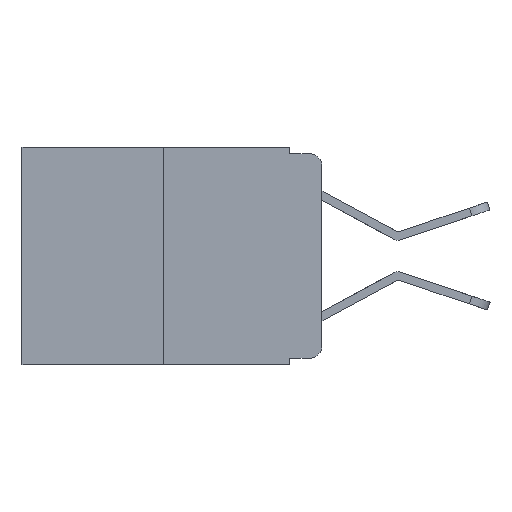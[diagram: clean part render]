
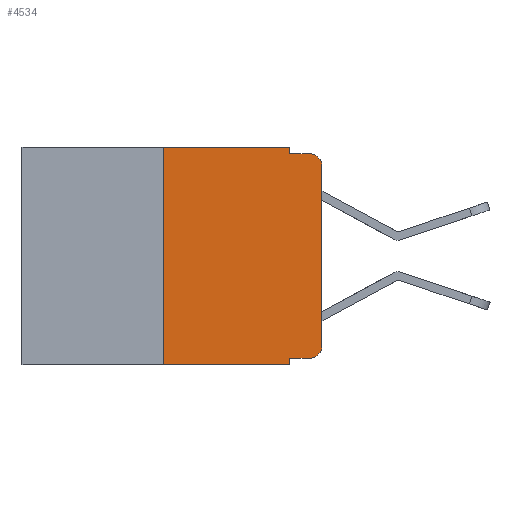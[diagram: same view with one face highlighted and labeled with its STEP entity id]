
A CAD part, left-side view. The second image highlights one B-rep face of the part: STEP entity #4534.
In plain terms, the highlighted planar face has unit normal (-1, 0, 0).
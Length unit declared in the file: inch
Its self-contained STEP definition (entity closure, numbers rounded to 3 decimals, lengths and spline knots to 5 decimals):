
#170 = VECTOR ( 'NONE', #7346, 39.37008 ) ;
#396 = CARTESIAN_POINT ( 'NONE',  ( 0., 0.051, -0.01 ) ) ;
#484 = DIRECTION ( 'NONE',  ( 0., 0., -1. ) ) ;
#607 = LINE ( 'NONE', #7649, #4637 ) ;
#1021 = EDGE_LOOP ( 'NONE', ( #7943, #7743, #6263, #6348, #7878, #4430, #2256, #4209, #5686, #8690 ) ) ;
#1067 = DIRECTION ( 'NONE',  ( 0., -1., 0. ) ) ;
#1153 = VECTOR ( 'NONE', #1067, 39.37008 ) ;
#1250 = LINE ( 'NONE', #10787, #1153 ) ;
#1366 = CARTESIAN_POINT ( 'NONE',  ( 0., 0.473, 0. ) ) ;
#1477 = CARTESIAN_POINT ( 'NONE',  ( 0., 0.051, 0. ) ) ;
#1480 = VECTOR ( 'NONE', #3447, 39.37008 ) ;
#1621 = CARTESIAN_POINT ( 'NONE',  ( 0., 0.25, -0.343 ) ) ;
#1725 = PLANE ( 'NONE',  #6695 ) ;
#1991 = EDGE_CURVE ( 'NONE', #6588, #9269, #6176, .T. ) ;
#2256 = ORIENTED_EDGE ( 'NONE', *, *, #5963, .T. ) ;
#2445 = CARTESIAN_POINT ( 'NONE',  ( 0., 0.02, -0.03 ) ) ;
#2461 = VECTOR ( 'NONE', #8202, 39.37008 ) ;
#3394 = DIRECTION ( 'NONE',  ( 1., 0., 0. ) ) ;
#3447 = DIRECTION ( 'NONE',  ( 0., -1., 0. ) ) ;
#3493 = CARTESIAN_POINT ( 'NONE',  ( 0., 0.25, 0. ) ) ;
#3704 = AXIS2_PLACEMENT_3D ( 'NONE', #7053, #9629, #11467 ) ;
#3713 = VERTEX_POINT ( 'NONE', #396 ) ;
#3797 = CARTESIAN_POINT ( 'NONE',  ( 0., 0.051, -0.333 ) ) ;
#3805 = DIRECTION ( 'NONE',  ( 0., 0., 1. ) ) ;
#3900 = CIRCLE ( 'NONE', #3704, 0.02 ) ;
#3915 = DIRECTION ( 'NONE',  ( 0., 0., 1. ) ) ;
#4080 = LINE ( 'NONE', #1477, #5767 ) ;
#4128 = CARTESIAN_POINT ( 'NONE',  ( 0., 0.02, -0.01 ) ) ;
#4209 = ORIENTED_EDGE ( 'NONE', *, *, #9113, .F. ) ;
#4430 = ORIENTED_EDGE ( 'NONE', *, *, #5489, .F. ) ;
#4435 = CARTESIAN_POINT ( 'NONE',  ( 0., 0.051, -0.01 ) ) ;
#4505 = EDGE_CURVE ( 'NONE', #3713, #9269, #9638, .T. ) ;
#4534 = ADVANCED_FACE ( 'NONE', ( #7171 ), #1725, .F. ) ;
#4637 = VECTOR ( 'NONE', #3915, 39.37008 ) ;
#4717 = EDGE_CURVE ( 'NONE', #8945, #5962, #9343, .T. ) ;
#5061 = DIRECTION ( 'NONE',  ( -1., 0., 0. ) ) ;
#5208 = VERTEX_POINT ( 'NONE', #1621 ) ;
#5489 = EDGE_CURVE ( 'NONE', #5208, #8945, #9243, .T. ) ;
#5626 = AXIS2_PLACEMENT_3D ( 'NONE', #2445, #5061, #7573 ) ;
#5686 = ORIENTED_EDGE ( 'NONE', *, *, #10804, .T. ) ;
#5767 = VECTOR ( 'NONE', #484, 39.37008 ) ;
#5785 = VERTEX_POINT ( 'NONE', #11475 ) ;
#5962 = VERTEX_POINT ( 'NONE', #10102 ) ;
#5963 = EDGE_CURVE ( 'NONE', #5208, #6996, #1250, .T. ) ;
#6176 = CIRCLE ( 'NONE', #5626, 0.02 ) ;
#6263 = ORIENTED_EDGE ( 'NONE', *, *, #4505, .F. ) ;
#6348 = ORIENTED_EDGE ( 'NONE', *, *, #8697, .F. ) ;
#6588 = VERTEX_POINT ( 'NONE', #9560 ) ;
#6695 = AXIS2_PLACEMENT_3D ( 'NONE', #10729, #3394, #8821 ) ;
#6996 = VERTEX_POINT ( 'NONE', #11272 ) ;
#7053 = CARTESIAN_POINT ( 'NONE',  ( 0., 0.02, -0.313 ) ) ;
#7171 = FACE_OUTER_BOUND ( 'NONE', #1021, .T. ) ;
#7205 = LINE ( 'NONE', #10766, #2461 ) ;
#7289 = CARTESIAN_POINT ( 'NONE',  ( 0., 0.051, 0. ) ) ;
#7346 = DIRECTION ( 'NONE',  ( 0., 0., -1. ) ) ;
#7453 = VECTOR ( 'NONE', #9281, 39.37008 ) ;
#7573 = DIRECTION ( 'NONE',  ( 0., 0., -1. ) ) ;
#7649 = CARTESIAN_POINT ( 'NONE',  ( 0., 0., 0. ) ) ;
#7743 = ORIENTED_EDGE ( 'NONE', *, *, #1991, .T. ) ;
#7878 = ORIENTED_EDGE ( 'NONE', *, *, #4717, .F. ) ;
#7943 = ORIENTED_EDGE ( 'NONE', *, *, #8761, .T. ) ;
#8202 = DIRECTION ( 'NONE',  ( 0., -1., 0. ) ) ;
#8648 = VERTEX_POINT ( 'NONE', #3797 ) ;
#8690 = ORIENTED_EDGE ( 'NONE', *, *, #8912, .T. ) ;
#8697 = EDGE_CURVE ( 'NONE', #5962, #3713, #4080, .T. ) ;
#8761 = EDGE_CURVE ( 'NONE', #9407, #6588, #607, .T. ) ;
#8821 = DIRECTION ( 'NONE',  ( 0., 0., -1. ) ) ;
#8912 = EDGE_CURVE ( 'NONE', #5785, #9407, #3900, .T. ) ;
#8945 = VERTEX_POINT ( 'NONE', #3493 ) ;
#9090 = LINE ( 'NONE', #7289, #170 ) ;
#9113 = EDGE_CURVE ( 'NONE', #8648, #6996, #9090, .T. ) ;
#9243 = LINE ( 'NONE', #11043, #11344 ) ;
#9269 = VERTEX_POINT ( 'NONE', #4128 ) ;
#9281 = DIRECTION ( 'NONE',  ( 0., -1., 0. ) ) ;
#9343 = LINE ( 'NONE', #1366, #7453 ) ;
#9407 = VERTEX_POINT ( 'NONE', #11284 ) ;
#9560 = CARTESIAN_POINT ( 'NONE',  ( 0., 0., -0.03 ) ) ;
#9629 = DIRECTION ( 'NONE',  ( -1., 0., 0. ) ) ;
#9638 = LINE ( 'NONE', #4435, #1480 ) ;
#10102 = CARTESIAN_POINT ( 'NONE',  ( 0., 0.051, 0. ) ) ;
#10729 = CARTESIAN_POINT ( 'NONE',  ( 0., 0.473, 0. ) ) ;
#10766 = CARTESIAN_POINT ( 'NONE',  ( 0., 0.051, -0.333 ) ) ;
#10787 = CARTESIAN_POINT ( 'NONE',  ( 0., 0.473, -0.343 ) ) ;
#10804 = EDGE_CURVE ( 'NONE', #8648, #5785, #7205, .T. ) ;
#11043 = CARTESIAN_POINT ( 'NONE',  ( 0., 0.25, 0. ) ) ;
#11272 = CARTESIAN_POINT ( 'NONE',  ( 0., 0.051, -0.343 ) ) ;
#11284 = CARTESIAN_POINT ( 'NONE',  ( 0., 0., -0.313 ) ) ;
#11344 = VECTOR ( 'NONE', #3805, 39.37008 ) ;
#11467 = DIRECTION ( 'NONE',  ( 0., 0., -1. ) ) ;
#11475 = CARTESIAN_POINT ( 'NONE',  ( 0., 0.02, -0.333 ) ) ;
